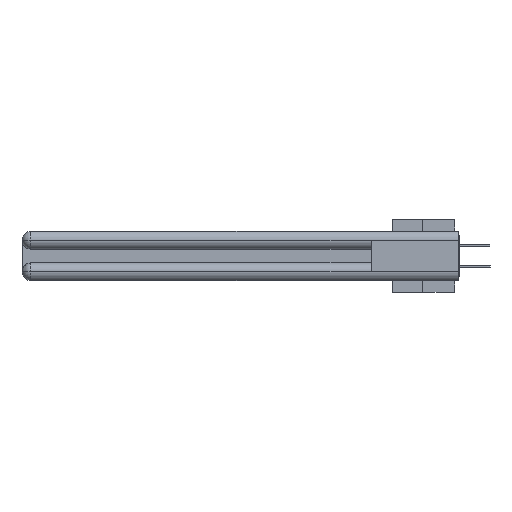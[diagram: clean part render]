
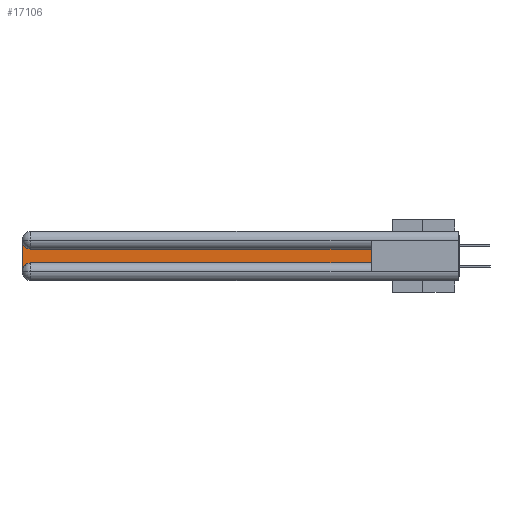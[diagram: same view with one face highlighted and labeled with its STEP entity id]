
A CAD part, left-side view. The second image highlights one B-rep face of the part: STEP entity #17106.
In plain terms, the highlighted planar face has unit normal (-1, 0, 0).
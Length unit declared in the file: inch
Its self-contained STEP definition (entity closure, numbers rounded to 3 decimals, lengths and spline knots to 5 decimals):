
#219 = ORIENTED_EDGE ( 'NONE', *, *, #16943, .T. ) ;
#3020 = CIRCLE ( 'NONE', #29646, 0.06 ) ;
#3299 = CARTESIAN_POINT ( 'NONE',  ( 0.075, 0.6, -0.1225 ) ) ;
#4279 = ORIENTED_EDGE ( 'NONE', *, *, #33995, .T. ) ;
#4569 = DIRECTION ( 'NONE',  ( 0., 0., -1. ) ) ;
#5117 = DIRECTION ( 'NONE',  ( 0., -1., 0. ) ) ;
#5241 = VECTOR ( 'NONE', #37409, 39.37008 ) ;
#5437 = DIRECTION ( 'NONE',  ( 0., 0., -1. ) ) ;
#5868 = CARTESIAN_POINT ( 'NONE',  ( 0.075, 2.94, -0.0625 ) ) ;
#5932 = VERTEX_POINT ( 'NONE', #15674 ) ;
#9588 = LINE ( 'NONE', #32983, #29877 ) ;
#10930 = LINE ( 'NONE', #33479, #5241 ) ;
#13555 = VERTEX_POINT ( 'NONE', #27385 ) ;
#13653 = CARTESIAN_POINT ( 'NONE',  ( 0.075, 3., -0.0625 ) ) ;
#14198 = DIRECTION ( 'NONE',  ( 1., 0., 0. ) ) ;
#15047 = AXIS2_PLACEMENT_3D ( 'NONE', #41095, #28074, #37755 ) ;
#15099 = EDGE_LOOP ( 'NONE', ( #26844, #36536, #219, #4279, #39624, #15835 ) ) ;
#15674 = CARTESIAN_POINT ( 'NONE',  ( 0.075, 3., -0.2775 ) ) ;
#15835 = ORIENTED_EDGE ( 'NONE', *, *, #26886, .T. ) ;
#16011 = EDGE_CURVE ( 'NONE', #24985, #19351, #42017, .T. ) ;
#16943 = EDGE_CURVE ( 'NONE', #19351, #5932, #9588, .T. ) ;
#17106 = ADVANCED_FACE ( 'NONE', ( #33051 ), #31021, .F. ) ;
#19351 = VERTEX_POINT ( 'NONE', #13653 ) ;
#21774 = VERTEX_POINT ( 'NONE', #32859 ) ;
#22220 = EDGE_CURVE ( 'NONE', #38405, #21774, #29452, .T. ) ;
#23129 = CARTESIAN_POINT ( 'NONE',  ( 0.075, 2.94, -0.1225 ) ) ;
#24985 = VERTEX_POINT ( 'NONE', #23129 ) ;
#26813 = VECTOR ( 'NONE', #5117, 39.37008 ) ;
#26844 = ORIENTED_EDGE ( 'NONE', *, *, #33893, .T. ) ;
#26886 = EDGE_CURVE ( 'NONE', #21774, #13555, #10930, .T. ) ;
#27385 = CARTESIAN_POINT ( 'NONE',  ( 0.075, 0.6, -0.1225 ) ) ;
#28074 = DIRECTION ( 'NONE',  ( 1., 0., 0. ) ) ;
#29452 = LINE ( 'NONE', #35307, #26813 ) ;
#29646 = AXIS2_PLACEMENT_3D ( 'NONE', #31070, #14198, #4569 ) ;
#29877 = VECTOR ( 'NONE', #35626, 39.37008 ) ;
#30086 = DIRECTION ( 'NONE',  ( 0., 1., 0. ) ) ;
#31021 = PLANE ( 'NONE',  #15047 ) ;
#31070 = CARTESIAN_POINT ( 'NONE',  ( 0.075, 2.94, -0.2775 ) ) ;
#32552 = DIRECTION ( 'NONE',  ( 1., 0., 0. ) ) ;
#32859 = CARTESIAN_POINT ( 'NONE',  ( 0.075, 0.6, -0.2175 ) ) ;
#32983 = CARTESIAN_POINT ( 'NONE',  ( 0.075, 3., -0.2175 ) ) ;
#33051 = FACE_OUTER_BOUND ( 'NONE', #15099, .T. ) ;
#33479 = CARTESIAN_POINT ( 'NONE',  ( 0.075, 0.6, -0.2175 ) ) ;
#33893 = EDGE_CURVE ( 'NONE', #13555, #24985, #35935, .T. ) ;
#33995 = EDGE_CURVE ( 'NONE', #5932, #38405, #3020, .T. ) ;
#35307 = CARTESIAN_POINT ( 'NONE',  ( 0.075, 0.6, -0.2175 ) ) ;
#35626 = DIRECTION ( 'NONE',  ( 0., 0., -1. ) ) ;
#35935 = LINE ( 'NONE', #3299, #36441 ) ;
#36284 = AXIS2_PLACEMENT_3D ( 'NONE', #5868, #32552, #5437 ) ;
#36441 = VECTOR ( 'NONE', #30086, 39.37008 ) ;
#36536 = ORIENTED_EDGE ( 'NONE', *, *, #16011, .T. ) ;
#37409 = DIRECTION ( 'NONE',  ( 0., 0., 1. ) ) ;
#37661 = CARTESIAN_POINT ( 'NONE',  ( 0.075, 2.94, -0.2175 ) ) ;
#37755 = DIRECTION ( 'NONE',  ( 0., 0., -1. ) ) ;
#38405 = VERTEX_POINT ( 'NONE', #37661 ) ;
#39624 = ORIENTED_EDGE ( 'NONE', *, *, #22220, .T. ) ;
#41095 = CARTESIAN_POINT ( 'NONE',  ( 0.075, 3., -0.1225 ) ) ;
#42017 = CIRCLE ( 'NONE', #36284, 0.06 ) ;
